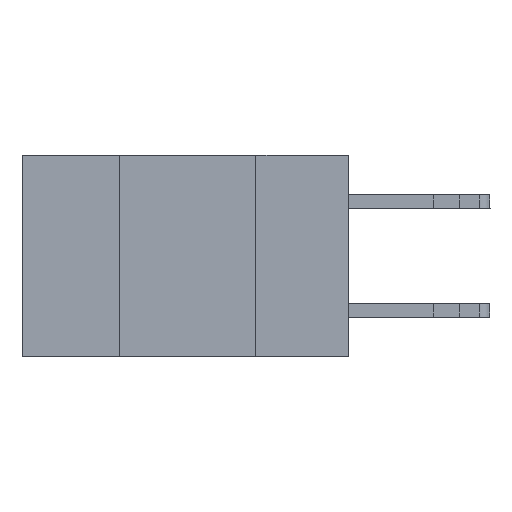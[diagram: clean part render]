
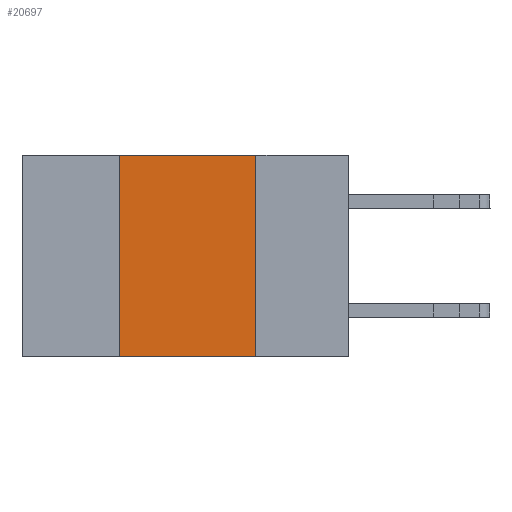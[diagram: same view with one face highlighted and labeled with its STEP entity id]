
A CAD part, left-side view. The second image highlights one B-rep face of the part: STEP entity #20697.
In plain terms, the highlighted planar face has unit normal (-1, 0, 0).
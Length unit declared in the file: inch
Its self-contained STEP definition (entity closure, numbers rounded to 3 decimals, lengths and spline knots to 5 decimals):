
#309 = VECTOR ( 'NONE', #2412, 39.37008 ) ;
#1823 = EDGE_LOOP ( 'NONE', ( #6261, #17031, #16480, #16178 ) ) ;
#2412 = DIRECTION ( 'NONE',  ( 0., -1., 0. ) ) ;
#2534 = CARTESIAN_POINT ( 'NONE',  ( 0., 0.6, 0. ) ) ;
#3852 = VERTEX_POINT ( 'NONE', #6644 ) ;
#4253 = VECTOR ( 'NONE', #13842, 39.37008 ) ;
#5441 = DIRECTION ( 'NONE',  ( 0., 0., 1. ) ) ;
#5713 = CARTESIAN_POINT ( 'NONE',  ( 0., 0.6, -0.37 ) ) ;
#6261 = ORIENTED_EDGE ( 'NONE', *, *, #16622, .F. ) ;
#6644 = CARTESIAN_POINT ( 'NONE',  ( 0., 0.17, -0.37 ) ) ;
#6964 = CARTESIAN_POINT ( 'NONE',  ( 0., 0.17, 0. ) ) ;
#8124 = VECTOR ( 'NONE', #5441, 39.37008 ) ;
#8292 = VECTOR ( 'NONE', #15023, 39.37008 ) ;
#8381 = DIRECTION ( 'NONE',  ( 1., 0., 0. ) ) ;
#8614 = CARTESIAN_POINT ( 'NONE',  ( 0., 0.42, 0. ) ) ;
#8975 = VERTEX_POINT ( 'NONE', #9617 ) ;
#9285 = EDGE_CURVE ( 'NONE', #11895, #8975, #11378, .T. ) ;
#9517 = CARTESIAN_POINT ( 'NONE',  ( 0., 0.42, -0.37 ) ) ;
#9617 = CARTESIAN_POINT ( 'NONE',  ( 0., 0.42, 0. ) ) ;
#10530 = EDGE_CURVE ( 'NONE', #8975, #10740, #12334, .T. ) ;
#10740 = VERTEX_POINT ( 'NONE', #19052 ) ;
#11378 = LINE ( 'NONE', #8614, #8124 ) ;
#11895 = VERTEX_POINT ( 'NONE', #9517 ) ;
#12334 = LINE ( 'NONE', #2534, #4253 ) ;
#13164 = PLANE ( 'NONE',  #17061 ) ;
#13306 = LINE ( 'NONE', #5713, #309 ) ;
#13842 = DIRECTION ( 'NONE',  ( 0., -1., 0. ) ) ;
#15023 = DIRECTION ( 'NONE',  ( 0., 0., -1. ) ) ;
#16178 = ORIENTED_EDGE ( 'NONE', *, *, #16768, .T. ) ;
#16319 = LINE ( 'NONE', #6964, #8292 ) ;
#16382 = CARTESIAN_POINT ( 'NONE',  ( 0., 0.6, 0. ) ) ;
#16385 = FACE_OUTER_BOUND ( 'NONE', #1823, .T. ) ;
#16480 = ORIENTED_EDGE ( 'NONE', *, *, #9285, .F. ) ;
#16622 = EDGE_CURVE ( 'NONE', #10740, #3852, #16319, .T. ) ;
#16768 = EDGE_CURVE ( 'NONE', #11895, #3852, #13306, .T. ) ;
#17031 = ORIENTED_EDGE ( 'NONE', *, *, #10530, .F. ) ;
#17061 = AXIS2_PLACEMENT_3D ( 'NONE', #16382, #8381, #19558 ) ;
#19052 = CARTESIAN_POINT ( 'NONE',  ( 0., 0.17, 0. ) ) ;
#19558 = DIRECTION ( 'NONE',  ( 0., 0., -1. ) ) ;
#20697 = ADVANCED_FACE ( 'NONE', ( #16385 ), #13164, .F. ) ;
